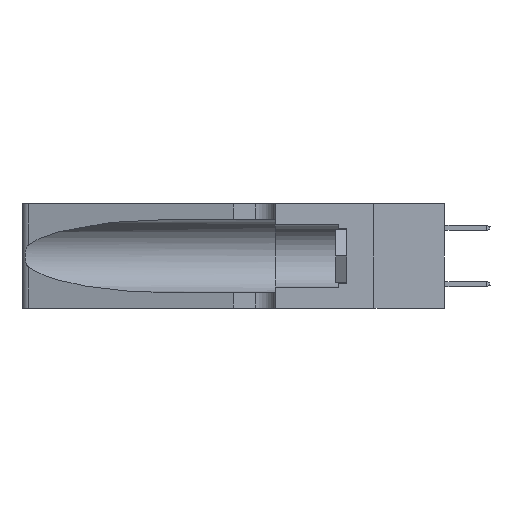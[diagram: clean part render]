
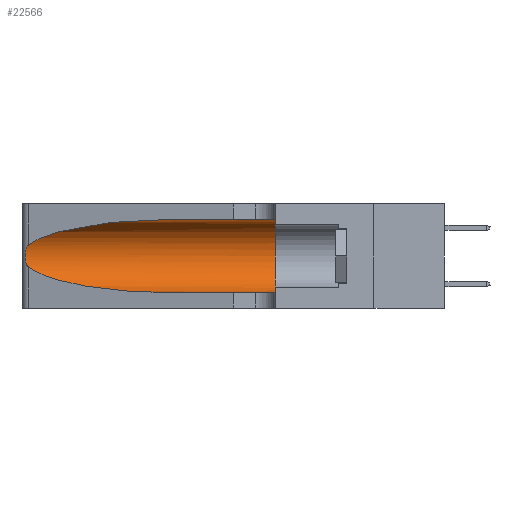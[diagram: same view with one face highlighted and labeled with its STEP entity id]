
A CAD part, left-side view. The second image highlights one B-rep face of the part: STEP entity #22566.
In plain terms, the highlighted cylindrical face has radius 3.308 mm (diameter 6.617 mm), a partial arc.
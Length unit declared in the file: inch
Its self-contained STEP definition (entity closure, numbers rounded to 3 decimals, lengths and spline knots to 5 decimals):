
#549 = CYLINDRICAL_SURFACE ( 'NONE', #16463, 0.13025 ) ;
#669 = CARTESIAN_POINT ( 'NONE',  ( 0.25487, 1.22718, 0.22369 ) ) ;
#1319 = CARTESIAN_POINT ( 'NONE',  ( 0.1305, 0.72297, 0.05475 ) ) ;
#3304 = CARTESIAN_POINT ( 'NONE',  ( 0.25787, 1.23484, 0.2124 ) ) ;
#4898 = VERTEX_POINT ( 'NONE', #12844 ) ;
#5327 = VERTEX_POINT ( 'NONE', #37058 ) ;
#6624 = CARTESIAN_POINT ( 'NONE',  ( 0.26018, 1.23835, 0.19895 ) ) ;
#7380 = CARTESIAN_POINT ( 'NONE',  ( 0.1305, 1.61858, 0.05475 ) ) ;
#9257 = ORIENTED_EDGE ( 'NONE', *, *, #41500, .T. ) ;
#9732 = CARTESIAN_POINT ( 'NONE',  ( 0.25487, 1.22718, 0.22369 ) ) ;
#9877 = CARTESIAN_POINT ( 'NONE',  ( 0.26075, 1.23896, 0.178 ) ) ;
#10574 = CARTESIAN_POINT ( 'NONE',  ( 0.25487, 1.22718, 0.22369 ) ) ;
#10630 = ORIENTED_EDGE ( 'NONE', *, *, #18119, .T. ) ;
#10995 = VERTEX_POINT ( 'NONE', #41403 ) ;
#12379 = EDGE_CURVE ( 'NONE', #12485, #40690, #18281, .T. ) ;
#12485 = VERTEX_POINT ( 'NONE', #10574 ) ;
#12656 = CARTESIAN_POINT ( 'NONE',  ( 0.1305, 1.61858, 0.31525 ) ) ;
#12844 = CARTESIAN_POINT ( 'NONE',  ( 0.1305, 0.35, 0.31525 ) ) ;
#13115 = CARTESIAN_POINT ( 'NONE',  ( 0.25856, 1.23593, 0.16098 ) ) ;
#13709 = CARTESIAN_POINT ( 'NONE',  ( 0.1305, 0.72297, 0.31525 ) ) ;
#14326 = CARTESIAN_POINT ( 'NONE',  ( 0.2373, 1.15595, 0.08982 ) ) ;
#16334 = CARTESIAN_POINT ( 'NONE',  ( 0.25639, 1.23186, 0.15144 ) ) ;
#16463 = AXIS2_PLACEMENT_3D ( 'NONE', #36927, #40116, #27340 ) ;
#16843 = CARTESIAN_POINT ( 'NONE',  ( 0.1305, 0.35, 0.05475 ) ) ;
#17888 = CARTESIAN_POINT ( 'NONE',  ( 0.1305, 0.35, 0.185 ) ) ;
#18119 = EDGE_CURVE ( 'NONE', #5327, #24887, #22310, .T. ) ;
#18281 = B_SPLINE_CURVE_WITH_KNOTS ( 'NONE', 3,
 ( #9732, #41706, #19458, #3304, #25820, #6624, #29027, #9877, #32230, #13115, #35443, #16334, #38611, #19587 ),
 .UNSPECIFIED., .F., .F.,
 ( 4, 2, 2, 2, 2, 2, 4 ),
 ( 0., 0.00027, 0.00053, 0.00107, 0.0016, 0.00187, 0.00214 ),
 .UNSPECIFIED. ) ;
#19304 = CIRCLE ( 'NONE', #30221, 0.13025 ) ;
#19458 = CARTESIAN_POINT ( 'NONE',  ( 0.25639, 1.23184, 0.21858 ) ) ;
#19587 = CARTESIAN_POINT ( 'NONE',  ( 0.25487, 1.22718, 0.14631 ) ) ;
#20082 = EDGE_CURVE ( 'NONE', #10995, #4898, #31119, .T. ) ;
#20183 = CARTESIAN_POINT ( 'NONE',  ( 0.2373, 1.15595, 0.28018 ) ) ;
#20681 = VECTOR ( 'NONE', #22351, 39.37008 ) ;
#20806 = CARTESIAN_POINT ( 'NONE',  ( 0.18966, 0.96281, 0.05475 ) ) ;
#20985 = ORIENTED_EDGE ( 'NONE', *, *, #12379, .T. ) ;
#21123 = DIRECTION ( 'NONE',  ( 0., 0., 1. ) ) ;
#21315 = VECTOR ( 'NONE', #29773, 39.37008 ) ;
#22310 = LINE ( 'NONE', #7380, #21315 ) ;
#22351 = DIRECTION ( 'NONE',  ( 0., -1., 0. ) ) ;
#22529 = ORIENTED_EDGE ( 'NONE', *, *, #39220, .F. ) ;
#22566 = ADVANCED_FACE ( 'NONE', ( #34890 ), #549, .F. ) ;
#24397 = EDGE_LOOP ( 'NONE', ( #30502, #20985, #9257, #10630, #22529, #33920 ) ) ;
#24887 = VERTEX_POINT ( 'NONE', #16843 ) ;
#25820 = CARTESIAN_POINT ( 'NONE',  ( 0.25854, 1.2359, 0.20912 ) ) ;
#26938 =( BOUNDED_CURVE ( )  B_SPLINE_CURVE ( 3, ( #36618, #14326, #20806, #1319 ),
 .UNSPECIFIED., .F., .T. ) 
 B_SPLINE_CURVE_WITH_KNOTS ( ( 4, 4 ),
 ( 3.44316, 4.71239 ),
 .UNSPECIFIED. ) 
 CURVE ( )  GEOMETRIC_REPRESENTATION_ITEM ( )  RATIONAL_B_SPLINE_CURVE ( ( 1., 0.87, 0.87, 1. ) ) 
 REPRESENTATION_ITEM ( '' )  );
#27340 = DIRECTION ( 'NONE',  ( 0., 0., -1. ) ) ;
#29027 = CARTESIAN_POINT ( 'NONE',  ( 0.26075, 1.23896, 0.19203 ) ) ;
#29773 = DIRECTION ( 'NONE',  ( 0., -1., 0. ) ) ;
#30221 = AXIS2_PLACEMENT_3D ( 'NONE', #17888, #40140, #21123 ) ;
#30502 = ORIENTED_EDGE ( 'NONE', *, *, #34445, .T. ) ;
#31119 = LINE ( 'NONE', #12656, #20681 ) ;
#32230 = CARTESIAN_POINT ( 'NONE',  ( 0.26017, 1.23833, 0.17102 ) ) ;
#33920 = ORIENTED_EDGE ( 'NONE', *, *, #20082, .F. ) ;
#34354 =( BOUNDED_CURVE ( )  B_SPLINE_CURVE ( 3, ( #13709, #39217, #20183, #669 ),
 .UNSPECIFIED., .F., .F. ) 
 B_SPLINE_CURVE_WITH_KNOTS ( ( 4, 4 ),
 ( 1.5708, 2.84003 ),
 .UNSPECIFIED. ) 
 CURVE ( )  GEOMETRIC_REPRESENTATION_ITEM ( )  RATIONAL_B_SPLINE_CURVE ( ( 1., 0.87, 0.87, 1. ) ) 
 REPRESENTATION_ITEM ( '' )  );
#34445 = EDGE_CURVE ( 'NONE', #10995, #12485, #34354, .T. ) ;
#34890 = FACE_OUTER_BOUND ( 'NONE', #24397, .T. ) ;
#35443 = CARTESIAN_POINT ( 'NONE',  ( 0.25789, 1.23486, 0.15765 ) ) ;
#36618 = CARTESIAN_POINT ( 'NONE',  ( 0.25487, 1.22718, 0.14631 ) ) ;
#36927 = CARTESIAN_POINT ( 'NONE',  ( 0.1305, 1.61858, 0.185 ) ) ;
#37058 = CARTESIAN_POINT ( 'NONE',  ( 0.1305, 0.72297, 0.05475 ) ) ;
#38611 = CARTESIAN_POINT ( 'NONE',  ( 0.25555, 1.22993, 0.14849 ) ) ;
#39036 = CARTESIAN_POINT ( 'NONE',  ( 0.25487, 1.22718, 0.14631 ) ) ;
#39217 = CARTESIAN_POINT ( 'NONE',  ( 0.18966, 0.96281, 0.31525 ) ) ;
#39220 = EDGE_CURVE ( 'NONE', #4898, #24887, #19304, .T. ) ;
#40116 = DIRECTION ( 'NONE',  ( 0., -1., 0. ) ) ;
#40140 = DIRECTION ( 'NONE',  ( 0., 1., 0. ) ) ;
#40690 = VERTEX_POINT ( 'NONE', #39036 ) ;
#41403 = CARTESIAN_POINT ( 'NONE',  ( 0.1305, 0.72297, 0.31525 ) ) ;
#41500 = EDGE_CURVE ( 'NONE', #40690, #5327, #26938, .T. ) ;
#41706 = CARTESIAN_POINT ( 'NONE',  ( 0.25555, 1.22994, 0.2215 ) ) ;
